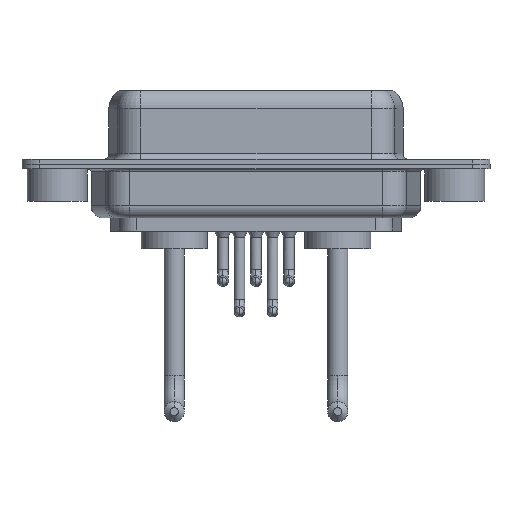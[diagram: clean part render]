
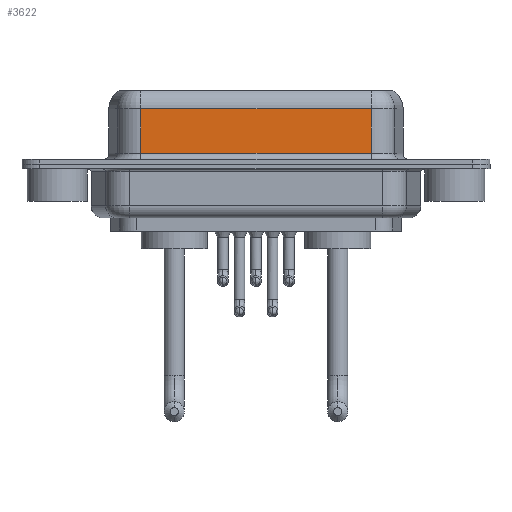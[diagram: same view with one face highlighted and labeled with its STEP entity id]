
A CAD part, front view. The second image highlights one B-rep face of the part: STEP entity #3622.
In plain terms, the highlighted planar face has unit normal (0, -1, 0).
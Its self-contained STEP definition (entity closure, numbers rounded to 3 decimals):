
#982 = CARTESIAN_POINT ( 'NONE',  ( 26.287, -3.95, 0.9 ) ) ;
#1653 = CARTESIAN_POINT ( 'NONE',  ( 26.287, -3.95, 0.9 ) ) ;
#1659 = AXIS2_PLACEMENT_3D ( 'NONE', #4954, #15661, #14125 ) ;
#2012 = DIRECTION ( 'NONE',  ( 0., 0., -1. ) ) ;
#3322 = VECTOR ( 'NONE', #3902, 1000. ) ;
#3622 = ADVANCED_FACE ( 'NONE', ( #9063 ), #3844, .F. ) ;
#3844 = PLANE ( 'NONE',  #1659 ) ;
#3892 = VECTOR ( 'NONE', #10495, 1000. ) ;
#3902 = DIRECTION ( 'NONE',  ( 1., 0., 0. ) ) ;
#3957 = EDGE_CURVE ( 'NONE', #13162, #4165, #11525, .T. ) ;
#4165 = VERTEX_POINT ( 'NONE', #1653 ) ;
#4560 = CARTESIAN_POINT ( 'NONE',  ( 26.287, -3.95, 4.65 ) ) ;
#4748 = LINE ( 'NONE', #14168, #15494 ) ;
#4954 = CARTESIAN_POINT ( 'NONE',  ( 26.287, -3.95, 6.4 ) ) ;
#5199 = EDGE_CURVE ( 'NONE', #14950, #4165, #8786, .T. ) ;
#5274 = ORIENTED_EDGE ( 'NONE', *, *, #13772, .T. ) ;
#5281 = LINE ( 'NONE', #15640, #3892 ) ;
#5306 = EDGE_CURVE ( 'NONE', #13266, #13162, #5281, .T. ) ;
#6487 = EDGE_LOOP ( 'NONE', ( #9237, #5274, #8708, #13817 ) ) ;
#6767 = CARTESIAN_POINT ( 'NONE',  ( 7.013, -3.95, 0.9 ) ) ;
#7321 = CARTESIAN_POINT ( 'NONE',  ( 26.287, -3.95, 6.4 ) ) ;
#8708 = ORIENTED_EDGE ( 'NONE', *, *, #5306, .T. ) ;
#8767 = DIRECTION ( 'NONE',  ( -1., 0., 0. ) ) ;
#8786 = LINE ( 'NONE', #7321, #15109 ) ;
#9063 = FACE_OUTER_BOUND ( 'NONE', #6487, .T. ) ;
#9237 = ORIENTED_EDGE ( 'NONE', *, *, #5199, .F. ) ;
#10495 = DIRECTION ( 'NONE',  ( 0., 0., -1. ) ) ;
#10624 = CARTESIAN_POINT ( 'NONE',  ( 7.013, -3.95, 4.65 ) ) ;
#11525 = LINE ( 'NONE', #982, #3322 ) ;
#13162 = VERTEX_POINT ( 'NONE', #6767 ) ;
#13266 = VERTEX_POINT ( 'NONE', #10624 ) ;
#13772 = EDGE_CURVE ( 'NONE', #14950, #13266, #4748, .T. ) ;
#13817 = ORIENTED_EDGE ( 'NONE', *, *, #3957, .T. ) ;
#14125 = DIRECTION ( 'NONE',  ( 0., 0., 1. ) ) ;
#14168 = CARTESIAN_POINT ( 'NONE',  ( 26.287, -3.95, 4.65 ) ) ;
#14950 = VERTEX_POINT ( 'NONE', #4560 ) ;
#15109 = VECTOR ( 'NONE', #2012, 1000. ) ;
#15494 = VECTOR ( 'NONE', #8767, 1000. ) ;
#15640 = CARTESIAN_POINT ( 'NONE',  ( 7.013, -3.95, 6.4 ) ) ;
#15661 = DIRECTION ( 'NONE',  ( 0., 1., 0. ) ) ;
